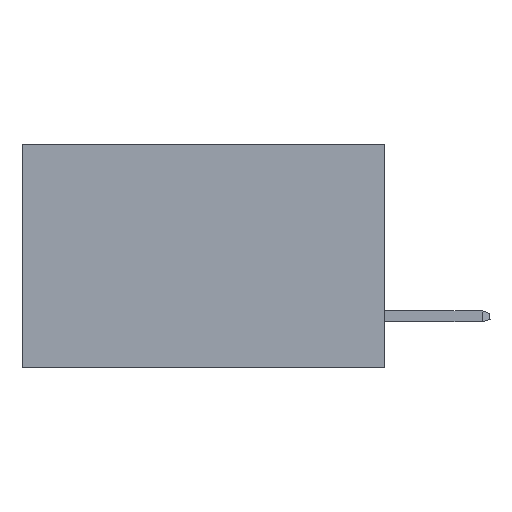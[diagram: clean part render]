
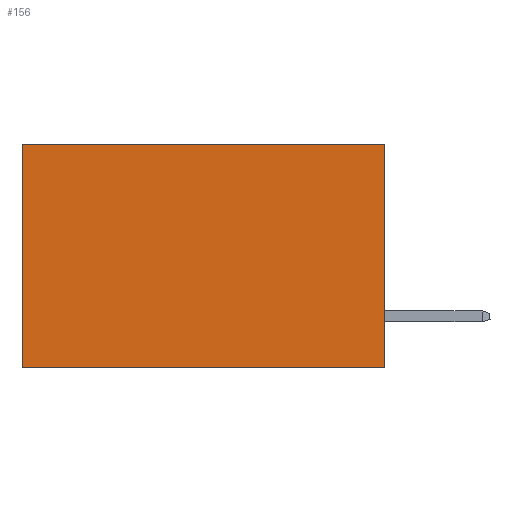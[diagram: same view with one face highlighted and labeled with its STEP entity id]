
A CAD part, left-side view. The second image highlights one B-rep face of the part: STEP entity #156.
In plain terms, the highlighted planar face has unit normal (-1, 0, 0).
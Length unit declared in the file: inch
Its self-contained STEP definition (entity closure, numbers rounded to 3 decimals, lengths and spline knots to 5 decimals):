
#156 = ADVANCED_FACE ( 'NONE', ( #7891 ), #8149, .F. ) ;
#207 = ORIENTED_EDGE ( 'NONE', *, *, #6392, .T. ) ;
#398 = DIRECTION ( 'NONE',  ( 0., 1., 0. ) ) ;
#525 = CARTESIAN_POINT ( 'NONE',  ( 0.298, 0., -0.37 ) ) ;
#1044 = CARTESIAN_POINT ( 'NONE',  ( 0.298, 0., 0. ) ) ;
#1095 = VECTOR ( 'NONE', #3564, 39.37008 ) ;
#1753 = LINE ( 'NONE', #525, #3448 ) ;
#2013 = DIRECTION ( 'NONE',  ( 0., 0., -1. ) ) ;
#2572 = AXIS2_PLACEMENT_3D ( 'NONE', #4733, #4851, #2013 ) ;
#2591 = DIRECTION ( 'NONE',  ( 0., 0., -1. ) ) ;
#2915 = EDGE_CURVE ( 'NONE', #7580, #6846, #4049, .T. ) ;
#3294 = ORIENTED_EDGE ( 'NONE', *, *, #7790, .T. ) ;
#3448 = VECTOR ( 'NONE', #398, 39.37008 ) ;
#3478 = EDGE_LOOP ( 'NONE', ( #3294, #4708, #4760, #207 ) ) ;
#3564 = DIRECTION ( 'NONE',  ( 0., 1., 0. ) ) ;
#3724 = CARTESIAN_POINT ( 'NONE',  ( 0.298, 0., 0. ) ) ;
#4049 = LINE ( 'NONE', #1044, #8389 ) ;
#4498 = VERTEX_POINT ( 'NONE', #5234 ) ;
#4708 = ORIENTED_EDGE ( 'NONE', *, *, #6756, .F. ) ;
#4733 = CARTESIAN_POINT ( 'NONE',  ( 0.298, 0., 0. ) ) ;
#4760 = ORIENTED_EDGE ( 'NONE', *, *, #2915, .F. ) ;
#4851 = DIRECTION ( 'NONE',  ( 1., 0., 0. ) ) ;
#5158 = VECTOR ( 'NONE', #5690, 39.37008 ) ;
#5234 = CARTESIAN_POINT ( 'NONE',  ( 0.298, 0.6, 0. ) ) ;
#5554 = CARTESIAN_POINT ( 'NONE',  ( 0.298, 0.6, -0.37 ) ) ;
#5690 = DIRECTION ( 'NONE',  ( 0., 0., -1. ) ) ;
#6392 = EDGE_CURVE ( 'NONE', #7580, #4498, #6795, .T. ) ;
#6756 = EDGE_CURVE ( 'NONE', #6846, #6779, #1753, .T. ) ;
#6779 = VERTEX_POINT ( 'NONE', #5554 ) ;
#6795 = LINE ( 'NONE', #7010, #1095 ) ;
#6846 = VERTEX_POINT ( 'NONE', #7537 ) ;
#6993 = LINE ( 'NONE', #8442, #5158 ) ;
#7010 = CARTESIAN_POINT ( 'NONE',  ( 0.298, 0., 0. ) ) ;
#7537 = CARTESIAN_POINT ( 'NONE',  ( 0.298, 0., -0.37 ) ) ;
#7580 = VERTEX_POINT ( 'NONE', #3724 ) ;
#7790 = EDGE_CURVE ( 'NONE', #4498, #6779, #6993, .T. ) ;
#7891 = FACE_OUTER_BOUND ( 'NONE', #3478, .T. ) ;
#8149 = PLANE ( 'NONE',  #2572 ) ;
#8389 = VECTOR ( 'NONE', #2591, 39.37008 ) ;
#8442 = CARTESIAN_POINT ( 'NONE',  ( 0.298, 0.6, 0. ) ) ;
